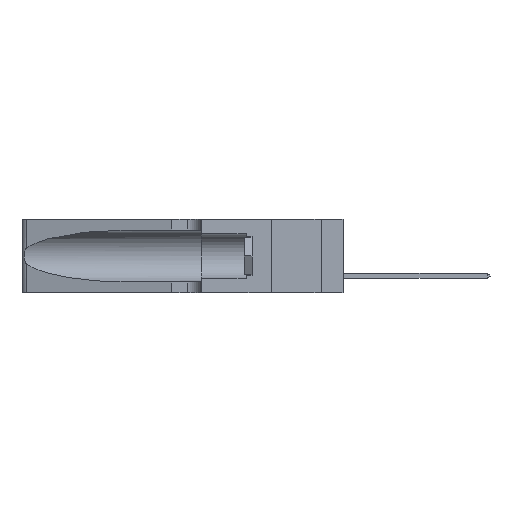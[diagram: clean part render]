
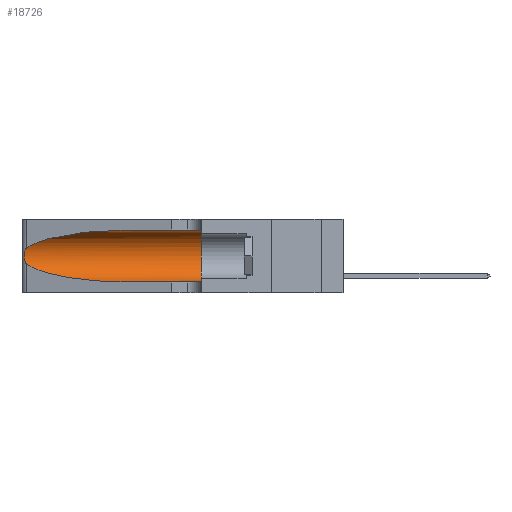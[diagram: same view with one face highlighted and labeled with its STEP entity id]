
A CAD part, left-side view. The second image highlights one B-rep face of the part: STEP entity #18726.
In plain terms, the highlighted cylindrical face has radius 3.308 mm (diameter 6.617 mm), a partial arc.
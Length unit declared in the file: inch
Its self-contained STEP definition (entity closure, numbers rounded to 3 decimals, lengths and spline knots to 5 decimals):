
#472 = CYLINDRICAL_SURFACE ( 'NONE', #13825, 0.13025 ) ;
#524 = CARTESIAN_POINT ( 'NONE',  ( 0.26017, 1.23833, 0.17102 ) ) ;
#1238 = EDGE_CURVE ( 'NONE', #33124, #16570, #5760, .T. ) ;
#2382 = EDGE_CURVE ( 'NONE', #25495, #27144, #15315, .T. ) ;
#2807 = ORIENTED_EDGE ( 'NONE', *, *, #14664, .F. ) ;
#3532 = DIRECTION ( 'NONE',  ( 0., -1., 0. ) ) ;
#3882 = CARTESIAN_POINT ( 'NONE',  ( 0.25487, 1.22718, 0.14631 ) ) ;
#4853 =( BOUNDED_CURVE ( )  B_SPLINE_CURVE ( 3, ( #3882, #32637, #35884, #30042 ),
 .UNSPECIFIED., .F., .F. ) 
 B_SPLINE_CURVE_WITH_KNOTS ( ( 4, 4 ),
 ( 3.44316, 4.71239 ),
 .UNSPECIFIED. ) 
 CURVE ( )  GEOMETRIC_REPRESENTATION_ITEM ( )  RATIONAL_B_SPLINE_CURVE ( ( 1., 0.87, 0.87, 1. ) ) 
 REPRESENTATION_ITEM ( '' )  );
#5760 =( BOUNDED_CURVE ( )  B_SPLINE_CURVE ( 3, ( #28910, #10610, #13246, #19556 ),
 .UNSPECIFIED., .F., .F. ) 
 B_SPLINE_CURVE_WITH_KNOTS ( ( 4, 4 ),
 ( 1.5708, 2.84003 ),
 .UNSPECIFIED. ) 
 CURVE ( )  GEOMETRIC_REPRESENTATION_ITEM ( )  RATIONAL_B_SPLINE_CURVE ( ( 1., 0.87, 0.87, 1. ) ) 
 REPRESENTATION_ITEM ( '' )  );
#7191 = DIRECTION ( 'NONE',  ( 0., 0., -1. ) ) ;
#7458 = DIRECTION ( 'NONE',  ( 0., -1., 0. ) ) ;
#8569 = FACE_OUTER_BOUND ( 'NONE', #11630, .T. ) ;
#8910 = CARTESIAN_POINT ( 'NONE',  ( 0.25789, 1.23486, 0.15765 ) ) ;
#9451 = EDGE_CURVE ( 'NONE', #33189, #27144, #12327, .T. ) ;
#10394 = CARTESIAN_POINT ( 'NONE',  ( 0.25487, 1.22718, 0.22369 ) ) ;
#10610 = CARTESIAN_POINT ( 'NONE',  ( 0.18966, 0.96281, 0.31525 ) ) ;
#10733 = CARTESIAN_POINT ( 'NONE',  ( 0.1305, 0.72297, 0.31525 ) ) ;
#10867 = CARTESIAN_POINT ( 'NONE',  ( 0.25639, 1.23184, 0.21858 ) ) ;
#11630 = EDGE_LOOP ( 'NONE', ( #29077, #13588, #12239, #30553, #18787, #2807 ) ) ;
#12239 = ORIENTED_EDGE ( 'NONE', *, *, #28760, .T. ) ;
#12327 = LINE ( 'NONE', #21490, #22768 ) ;
#12348 = VERTEX_POINT ( 'NONE', #33157 ) ;
#13190 = CARTESIAN_POINT ( 'NONE',  ( 0.1305, 0.35, 0.31525 ) ) ;
#13246 = CARTESIAN_POINT ( 'NONE',  ( 0.2373, 1.15595, 0.28018 ) ) ;
#13588 = ORIENTED_EDGE ( 'NONE', *, *, #19131, .T. ) ;
#13683 = DIRECTION ( 'NONE',  ( 0., 1., 0. ) ) ;
#13825 = AXIS2_PLACEMENT_3D ( 'NONE', #24742, #7458, #7191 ) ;
#13967 = CARTESIAN_POINT ( 'NONE',  ( 0.26075, 1.23896, 0.178 ) ) ;
#14664 = EDGE_CURVE ( 'NONE', #33124, #25495, #35214, .T. ) ;
#15315 = CIRCLE ( 'NONE', #15932, 0.13025 ) ;
#15932 = AXIS2_PLACEMENT_3D ( 'NONE', #22116, #13683, #22245 ) ;
#16570 = VERTEX_POINT ( 'NONE', #10394 ) ;
#16758 = CARTESIAN_POINT ( 'NONE',  ( 0.26018, 1.23835, 0.19895 ) ) ;
#18241 = CARTESIAN_POINT ( 'NONE',  ( 0.1305, 0.35, 0.05475 ) ) ;
#18726 = ADVANCED_FACE ( 'NONE', ( #8569 ), #472, .F. ) ;
#18787 = ORIENTED_EDGE ( 'NONE', *, *, #2382, .F. ) ;
#19131 = EDGE_CURVE ( 'NONE', #16570, #12348, #19781, .T. ) ;
#19556 = CARTESIAN_POINT ( 'NONE',  ( 0.25487, 1.22718, 0.22369 ) ) ;
#19781 = B_SPLINE_CURVE_WITH_KNOTS ( 'NONE', 3,
 ( #25167, #28043, #10867, #31479, #25875, #16758, #22528, #13967, #524, #20336, #8910, #26198, #28840, #34554 ),
 .UNSPECIFIED., .F., .F.,
 ( 4, 2, 2, 2, 2, 2, 4 ),
 ( 0., 0.00027, 0.00053, 0.00107, 0.0016, 0.00187, 0.00214 ),
 .UNSPECIFIED. ) ;
#20336 = CARTESIAN_POINT ( 'NONE',  ( 0.25856, 1.23593, 0.16098 ) ) ;
#20454 = CARTESIAN_POINT ( 'NONE',  ( 0.1305, 1.61858, 0.31525 ) ) ;
#21490 = CARTESIAN_POINT ( 'NONE',  ( 0.1305, 1.61858, 0.05475 ) ) ;
#22116 = CARTESIAN_POINT ( 'NONE',  ( 0.1305, 0.35, 0.185 ) ) ;
#22245 = DIRECTION ( 'NONE',  ( 0., 0., 1. ) ) ;
#22528 = CARTESIAN_POINT ( 'NONE',  ( 0.26075, 1.23896, 0.19203 ) ) ;
#22768 = VECTOR ( 'NONE', #35587, 39.37008 ) ;
#24742 = CARTESIAN_POINT ( 'NONE',  ( 0.1305, 1.61858, 0.185 ) ) ;
#25167 = CARTESIAN_POINT ( 'NONE',  ( 0.25487, 1.22718, 0.22369 ) ) ;
#25495 = VERTEX_POINT ( 'NONE', #13190 ) ;
#25875 = CARTESIAN_POINT ( 'NONE',  ( 0.25854, 1.2359, 0.20912 ) ) ;
#26198 = CARTESIAN_POINT ( 'NONE',  ( 0.25639, 1.23186, 0.15144 ) ) ;
#27144 = VERTEX_POINT ( 'NONE', #18241 ) ;
#27781 = CARTESIAN_POINT ( 'NONE',  ( 0.1305, 0.72297, 0.05475 ) ) ;
#28043 = CARTESIAN_POINT ( 'NONE',  ( 0.25555, 1.22994, 0.2215 ) ) ;
#28760 = EDGE_CURVE ( 'NONE', #12348, #33189, #4853, .T. ) ;
#28840 = CARTESIAN_POINT ( 'NONE',  ( 0.25555, 1.22993, 0.14849 ) ) ;
#28910 = CARTESIAN_POINT ( 'NONE',  ( 0.1305, 0.72297, 0.31525 ) ) ;
#29077 = ORIENTED_EDGE ( 'NONE', *, *, #1238, .T. ) ;
#30042 = CARTESIAN_POINT ( 'NONE',  ( 0.1305, 0.72297, 0.05475 ) ) ;
#30553 = ORIENTED_EDGE ( 'NONE', *, *, #9451, .T. ) ;
#31479 = CARTESIAN_POINT ( 'NONE',  ( 0.25787, 1.23484, 0.2124 ) ) ;
#32530 = VECTOR ( 'NONE', #3532, 39.37008 ) ;
#32637 = CARTESIAN_POINT ( 'NONE',  ( 0.2373, 1.15595, 0.08982 ) ) ;
#33124 = VERTEX_POINT ( 'NONE', #10733 ) ;
#33157 = CARTESIAN_POINT ( 'NONE',  ( 0.25487, 1.22718, 0.14631 ) ) ;
#33189 = VERTEX_POINT ( 'NONE', #27781 ) ;
#34554 = CARTESIAN_POINT ( 'NONE',  ( 0.25487, 1.22718, 0.14631 ) ) ;
#35214 = LINE ( 'NONE', #20454, #32530 ) ;
#35587 = DIRECTION ( 'NONE',  ( 0., -1., 0. ) ) ;
#35884 = CARTESIAN_POINT ( 'NONE',  ( 0.18966, 0.96281, 0.05475 ) ) ;
